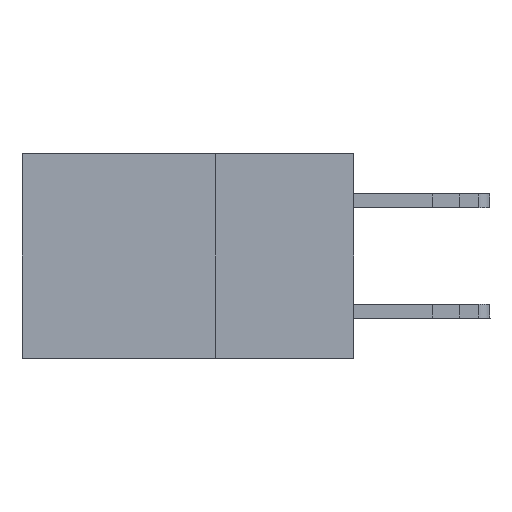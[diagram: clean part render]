
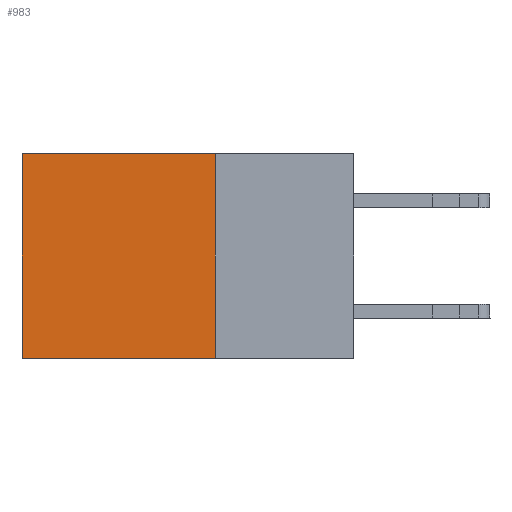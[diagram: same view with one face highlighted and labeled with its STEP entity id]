
A CAD part, left-side view. The second image highlights one B-rep face of the part: STEP entity #983.
In plain terms, the highlighted planar face has unit normal (-1, 0, 0).
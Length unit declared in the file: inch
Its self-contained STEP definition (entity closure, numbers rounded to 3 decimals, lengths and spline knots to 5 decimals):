
#983 = ADVANCED_FACE ( 'NONE', ( #23984 ), #21419, .F. ) ;
#3095 = EDGE_CURVE ( 'NONE', #18316, #19120, #13039, .T. ) ;
#3442 = CARTESIAN_POINT ( 'NONE',  ( 0.2875, 0.25, 0. ) ) ;
#3449 = EDGE_CURVE ( 'NONE', #6313, #18316, #3869, .T. ) ;
#3524 = DIRECTION ( 'NONE',  ( 0., 1., 0. ) ) ;
#3536 = VECTOR ( 'NONE', #16456, 39.37008 ) ;
#3869 = LINE ( 'NONE', #14433, #3536 ) ;
#5780 = EDGE_CURVE ( 'NONE', #6313, #24120, #20197, .T. ) ;
#6313 = VERTEX_POINT ( 'NONE', #15164 ) ;
#7550 = EDGE_CURVE ( 'NONE', #24120, #19120, #13232, .T. ) ;
#8354 = VECTOR ( 'NONE', #12387, 39.37008 ) ;
#10531 = CARTESIAN_POINT ( 'NONE',  ( 0.2875, 0.6, -0.37 ) ) ;
#10992 = AXIS2_PLACEMENT_3D ( 'NONE', #13564, #23339, #21262 ) ;
#11997 = ORIENTED_EDGE ( 'NONE', *, *, #5780, .T. ) ;
#12387 = DIRECTION ( 'NONE',  ( 0., 0., -1. ) ) ;
#12403 = VECTOR ( 'NONE', #16009, 39.37008 ) ;
#12758 = CARTESIAN_POINT ( 'NONE',  ( 0.2875, 0.25, -0.37 ) ) ;
#12920 = VECTOR ( 'NONE', #3524, 39.37008 ) ;
#13039 = LINE ( 'NONE', #13994, #12403 ) ;
#13232 = LINE ( 'NONE', #16222, #8354 ) ;
#13564 = CARTESIAN_POINT ( 'NONE',  ( 0.2875, 0.25, 0. ) ) ;
#13994 = CARTESIAN_POINT ( 'NONE',  ( 0.2875, 0.25, -0.37 ) ) ;
#14433 = CARTESIAN_POINT ( 'NONE',  ( 0.2875, 0.25, 0. ) ) ;
#15164 = CARTESIAN_POINT ( 'NONE',  ( 0.2875, 0.25, 0. ) ) ;
#16009 = DIRECTION ( 'NONE',  ( 0., 1., 0. ) ) ;
#16222 = CARTESIAN_POINT ( 'NONE',  ( 0.2875, 0.6, 0. ) ) ;
#16456 = DIRECTION ( 'NONE',  ( 0., 0., -1. ) ) ;
#17532 = EDGE_LOOP ( 'NONE', ( #22854, #17827, #20562, #11997 ) ) ;
#17827 = ORIENTED_EDGE ( 'NONE', *, *, #3095, .F. ) ;
#18316 = VERTEX_POINT ( 'NONE', #12758 ) ;
#19120 = VERTEX_POINT ( 'NONE', #10531 ) ;
#20197 = LINE ( 'NONE', #3442, #12920 ) ;
#20562 = ORIENTED_EDGE ( 'NONE', *, *, #3449, .F. ) ;
#21262 = DIRECTION ( 'NONE',  ( 0., 0., -1. ) ) ;
#21419 = PLANE ( 'NONE',  #10992 ) ;
#22854 = ORIENTED_EDGE ( 'NONE', *, *, #7550, .T. ) ;
#23339 = DIRECTION ( 'NONE',  ( 1., 0., 0. ) ) ;
#23984 = FACE_OUTER_BOUND ( 'NONE', #17532, .T. ) ;
#24120 = VERTEX_POINT ( 'NONE', #24474 ) ;
#24474 = CARTESIAN_POINT ( 'NONE',  ( 0.2875, 0.6, 0. ) ) ;
